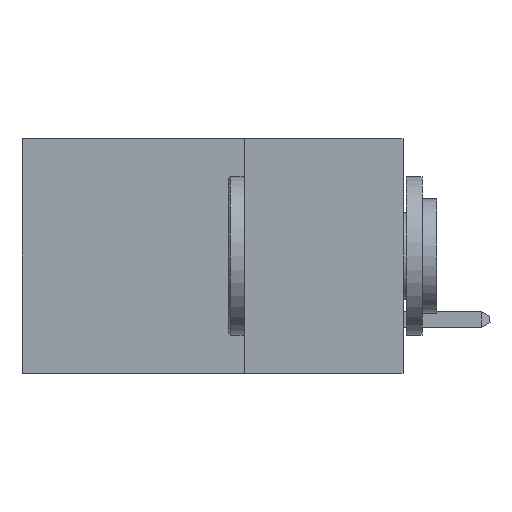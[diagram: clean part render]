
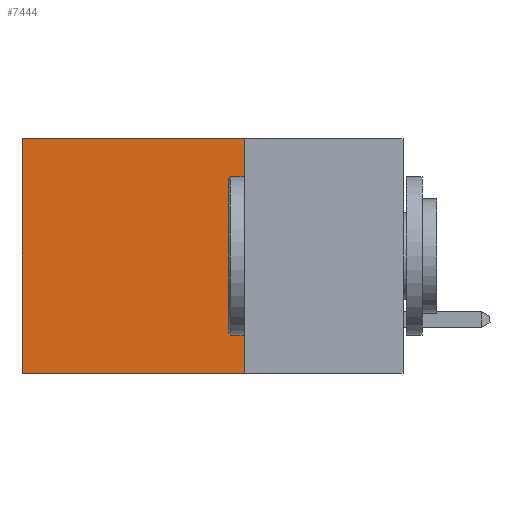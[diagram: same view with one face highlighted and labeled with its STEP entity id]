
A CAD part, left-side view. The second image highlights one B-rep face of the part: STEP entity #7444.
In plain terms, the highlighted planar face has unit normal (-1, 0, 0).
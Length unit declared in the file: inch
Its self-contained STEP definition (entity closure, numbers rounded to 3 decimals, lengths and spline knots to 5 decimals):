
#902 = CARTESIAN_POINT ( 'NONE',  ( 0.2875, 0.6, 0. ) ) ;
#926 = ORIENTED_EDGE ( 'NONE', *, *, #10566, .T. ) ;
#1806 = ORIENTED_EDGE ( 'NONE', *, *, #11948, .F. ) ;
#2416 = VERTEX_POINT ( 'NONE', #2657 ) ;
#2628 = EDGE_CURVE ( 'NONE', #3293, #5786, #8763, .T. ) ;
#2657 = CARTESIAN_POINT ( 'NONE',  ( 0.2875, 0.6, -0.37 ) ) ;
#3226 = ORIENTED_EDGE ( 'NONE', *, *, #2628, .F. ) ;
#3293 = VERTEX_POINT ( 'NONE', #8450 ) ;
#3393 = ORIENTED_EDGE ( 'NONE', *, *, #6912, .T. ) ;
#3689 = CARTESIAN_POINT ( 'NONE',  ( 0.2875, 0.25, 0. ) ) ;
#3902 = VERTEX_POINT ( 'NONE', #5641 ) ;
#4594 = LINE ( 'NONE', #902, #9542 ) ;
#4644 = DIRECTION ( 'NONE',  ( 0., 0., -1. ) ) ;
#4770 = CARTESIAN_POINT ( 'NONE',  ( 0.2875, 0.25, 0. ) ) ;
#4815 = DIRECTION ( 'NONE',  ( 0., 1., 0. ) ) ;
#5382 = LINE ( 'NONE', #11614, #7985 ) ;
#5641 = CARTESIAN_POINT ( 'NONE',  ( 0.2875, 0.6, 0. ) ) ;
#5670 = DIRECTION ( 'NONE',  ( 1., 0., 0. ) ) ;
#5786 = VERTEX_POINT ( 'NONE', #6441 ) ;
#6179 = VECTOR ( 'NONE', #4644, 39.37008 ) ;
#6441 = CARTESIAN_POINT ( 'NONE',  ( 0.2875, 0.25, -0.37 ) ) ;
#6568 = CARTESIAN_POINT ( 'NONE',  ( 0.2875, 0.25, 0. ) ) ;
#6912 = EDGE_CURVE ( 'NONE', #3293, #3902, #12420, .T. ) ;
#7229 = DIRECTION ( 'NONE',  ( 0., 0., -1. ) ) ;
#7444 = ADVANCED_FACE ( 'NONE', ( #11219 ), #11426, .F. ) ;
#7815 = AXIS2_PLACEMENT_3D ( 'NONE', #6568, #5670, #12360 ) ;
#7985 = VECTOR ( 'NONE', #4815, 39.37008 ) ;
#8450 = CARTESIAN_POINT ( 'NONE',  ( 0.2875, 0.25, 0. ) ) ;
#8763 = LINE ( 'NONE', #4770, #6179 ) ;
#9542 = VECTOR ( 'NONE', #7229, 39.37008 ) ;
#9667 = DIRECTION ( 'NONE',  ( 0., 1., 0. ) ) ;
#9930 = VECTOR ( 'NONE', #9667, 39.37008 ) ;
#10314 = EDGE_LOOP ( 'NONE', ( #926, #1806, #3226, #3393 ) ) ;
#10566 = EDGE_CURVE ( 'NONE', #3902, #2416, #4594, .T. ) ;
#11219 = FACE_OUTER_BOUND ( 'NONE', #10314, .T. ) ;
#11426 = PLANE ( 'NONE',  #7815 ) ;
#11614 = CARTESIAN_POINT ( 'NONE',  ( 0.2875, 0.25, -0.37 ) ) ;
#11948 = EDGE_CURVE ( 'NONE', #5786, #2416, #5382, .T. ) ;
#12360 = DIRECTION ( 'NONE',  ( 0., 0., -1. ) ) ;
#12420 = LINE ( 'NONE', #3689, #9930 ) ;
